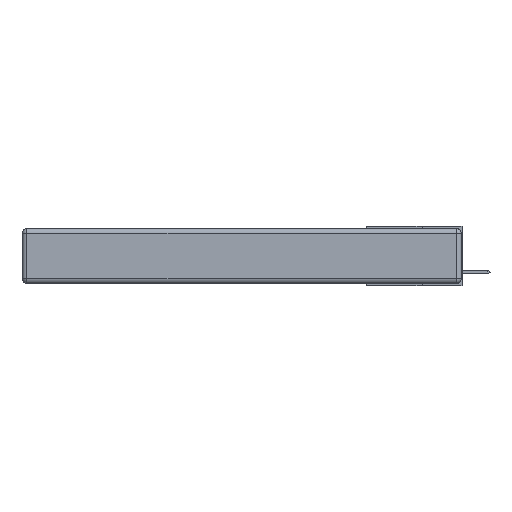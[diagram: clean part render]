
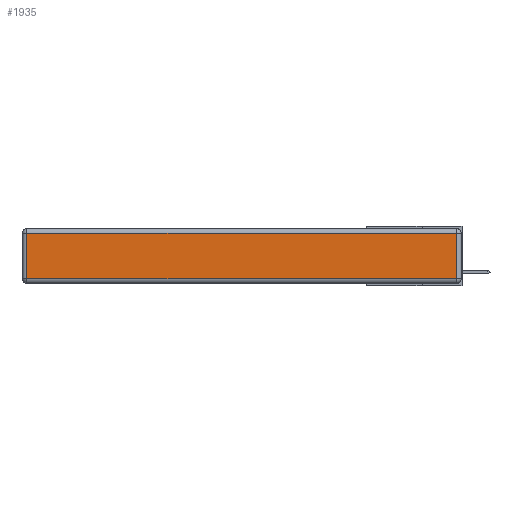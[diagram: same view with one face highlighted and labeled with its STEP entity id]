
A CAD part, left-side view. The second image highlights one B-rep face of the part: STEP entity #1935.
In plain terms, the highlighted planar face has unit normal (-1, 0, 0).
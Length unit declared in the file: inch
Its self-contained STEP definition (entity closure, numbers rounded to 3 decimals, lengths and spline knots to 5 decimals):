
#724 = LINE ( 'NONE', #9260, #10485 ) ;
#1271 = VERTEX_POINT ( 'NONE', #18157 ) ;
#1282 = EDGE_CURVE ( 'NONE', #5384, #3031, #724, .T. ) ;
#1935 = ADVANCED_FACE ( 'NONE', ( #19580 ), #7747, .T. ) ;
#3031 = VERTEX_POINT ( 'NONE', #20613 ) ;
#3528 = CARTESIAN_POINT ( 'NONE',  ( 0., 2.72, -0.343 ) ) ;
#4557 = ORIENTED_EDGE ( 'NONE', *, *, #10644, .T. ) ;
#5384 = VERTEX_POINT ( 'NONE', #16615 ) ;
#6133 = CARTESIAN_POINT ( 'NONE',  ( 0., 0.03, -0.313 ) ) ;
#6401 = LINE ( 'NONE', #7276, #15821 ) ;
#6612 = EDGE_CURVE ( 'NONE', #7813, #5384, #6401, .T. ) ;
#7276 = CARTESIAN_POINT ( 'NONE',  ( 0., 0.03, -0.343 ) ) ;
#7472 = ORIENTED_EDGE ( 'NONE', *, *, #21222, .T. ) ;
#7747 = PLANE ( 'NONE',  #10314 ) ;
#7813 = VERTEX_POINT ( 'NONE', #6133 ) ;
#9260 = CARTESIAN_POINT ( 'NONE',  ( 0., 2.75, -0.03 ) ) ;
#9443 = CARTESIAN_POINT ( 'NONE',  ( 0., 0., -0.343 ) ) ;
#9666 = DIRECTION ( 'NONE',  ( -1., 0., 0. ) ) ;
#10314 = AXIS2_PLACEMENT_3D ( 'NONE', #9443, #9666, #13243 ) ;
#10485 = VECTOR ( 'NONE', #11199, 39.37008 ) ;
#10596 = VECTOR ( 'NONE', #22513, 39.37008 ) ;
#10644 = EDGE_CURVE ( 'NONE', #3031, #1271, #11415, .T. ) ;
#11199 = DIRECTION ( 'NONE',  ( 0., 1., 0. ) ) ;
#11415 = LINE ( 'NONE', #3528, #10596 ) ;
#12241 = VECTOR ( 'NONE', #20742, 39.37008 ) ;
#13243 = DIRECTION ( 'NONE',  ( 0., 0., 1. ) ) ;
#14293 = ORIENTED_EDGE ( 'NONE', *, *, #6612, .T. ) ;
#15025 = EDGE_LOOP ( 'NONE', ( #7472, #14293, #19535, #4557 ) ) ;
#15821 = VECTOR ( 'NONE', #19435, 39.37008 ) ;
#16615 = CARTESIAN_POINT ( 'NONE',  ( 0., 0.03, -0.03 ) ) ;
#17169 = CARTESIAN_POINT ( 'NONE',  ( 0., 0., -0.313 ) ) ;
#17490 = LINE ( 'NONE', #17169, #12241 ) ;
#18157 = CARTESIAN_POINT ( 'NONE',  ( 0., 2.72, -0.313 ) ) ;
#19435 = DIRECTION ( 'NONE',  ( 0., 0., 1. ) ) ;
#19535 = ORIENTED_EDGE ( 'NONE', *, *, #1282, .T. ) ;
#19580 = FACE_OUTER_BOUND ( 'NONE', #15025, .T. ) ;
#20613 = CARTESIAN_POINT ( 'NONE',  ( 0., 2.72, -0.03 ) ) ;
#20742 = DIRECTION ( 'NONE',  ( 0., -1., 0. ) ) ;
#21222 = EDGE_CURVE ( 'NONE', #1271, #7813, #17490, .T. ) ;
#22513 = DIRECTION ( 'NONE',  ( 0., 0., -1. ) ) ;
